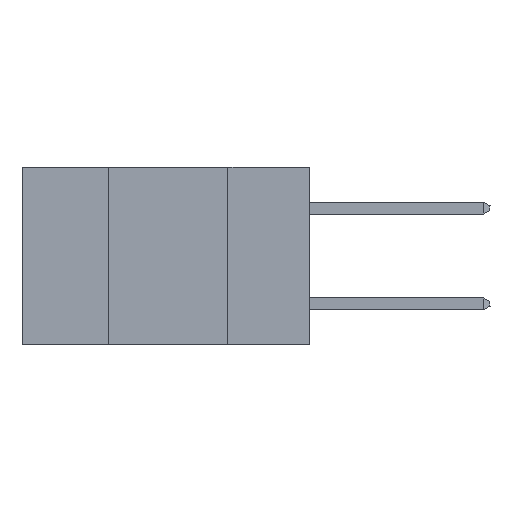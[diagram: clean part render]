
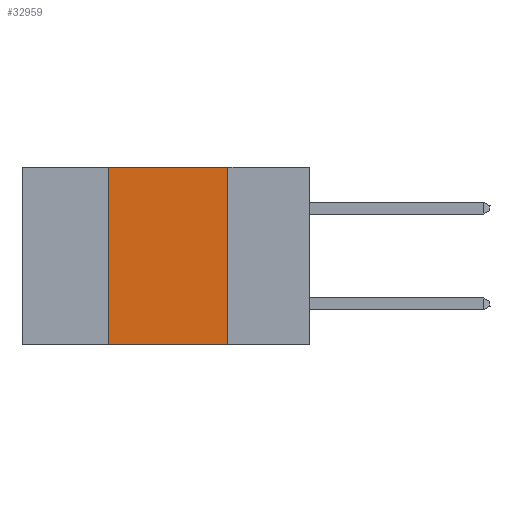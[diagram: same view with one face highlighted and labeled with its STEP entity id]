
A CAD part, left-side view. The second image highlights one B-rep face of the part: STEP entity #32959.
In plain terms, the highlighted planar face has unit normal (-1, 0, 0).
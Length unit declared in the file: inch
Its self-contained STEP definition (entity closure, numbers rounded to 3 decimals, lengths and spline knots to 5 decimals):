
#1785 = FACE_OUTER_BOUND ( 'NONE', #28149, .T. ) ;
#3760 = DIRECTION ( 'NONE',  ( 0., 0., 1. ) ) ;
#4637 = CARTESIAN_POINT ( 'NONE',  ( 0., 0.17, 0. ) ) ;
#5468 = DIRECTION ( 'NONE',  ( 0., -1., 0. ) ) ;
#6344 = CARTESIAN_POINT ( 'NONE',  ( 0., 0.6, -0.37 ) ) ;
#7379 = VERTEX_POINT ( 'NONE', #9560 ) ;
#9560 = CARTESIAN_POINT ( 'NONE',  ( 0., 0.42, 0. ) ) ;
#10012 = VERTEX_POINT ( 'NONE', #13973 ) ;
#13324 = CARTESIAN_POINT ( 'NONE',  ( 0., 0.42, -0.37 ) ) ;
#13857 = ORIENTED_EDGE ( 'NONE', *, *, #39722, .F. ) ;
#13973 = CARTESIAN_POINT ( 'NONE',  ( 0., 0.17, -0.37 ) ) ;
#15135 = CARTESIAN_POINT ( 'NONE',  ( 0., 0.42, 0. ) ) ;
#16659 = LINE ( 'NONE', #4637, #30544 ) ;
#18186 = LINE ( 'NONE', #23768, #26294 ) ;
#18479 = AXIS2_PLACEMENT_3D ( 'NONE', #45113, #23121, #43137 ) ;
#18833 = VERTEX_POINT ( 'NONE', #39176 ) ;
#21761 = VECTOR ( 'NONE', #3760, 39.37008 ) ;
#23121 = DIRECTION ( 'NONE',  ( 1., 0., 0. ) ) ;
#23596 = LINE ( 'NONE', #6344, #42101 ) ;
#23607 = EDGE_CURVE ( 'NONE', #18833, #10012, #16659, .T. ) ;
#23768 = CARTESIAN_POINT ( 'NONE',  ( 0., 0.6, 0. ) ) ;
#25855 = ORIENTED_EDGE ( 'NONE', *, *, #41841, .F. ) ;
#26294 = VECTOR ( 'NONE', #5468, 39.37008 ) ;
#28149 = EDGE_LOOP ( 'NONE', ( #29680, #25855, #13857, #33433 ) ) ;
#29680 = ORIENTED_EDGE ( 'NONE', *, *, #23607, .F. ) ;
#30544 = VECTOR ( 'NONE', #45440, 39.37008 ) ;
#32098 = DIRECTION ( 'NONE',  ( 0., -1., 0. ) ) ;
#32959 = ADVANCED_FACE ( 'NONE', ( #1785 ), #37883, .F. ) ;
#33433 = ORIENTED_EDGE ( 'NONE', *, *, #46192, .T. ) ;
#37883 = PLANE ( 'NONE',  #18479 ) ;
#39176 = CARTESIAN_POINT ( 'NONE',  ( 0., 0.17, 0. ) ) ;
#39722 = EDGE_CURVE ( 'NONE', #46052, #7379, #41415, .T. ) ;
#41415 = LINE ( 'NONE', #15135, #21761 ) ;
#41841 = EDGE_CURVE ( 'NONE', #7379, #18833, #18186, .T. ) ;
#42101 = VECTOR ( 'NONE', #32098, 39.37008 ) ;
#43137 = DIRECTION ( 'NONE',  ( 0., 0., -1. ) ) ;
#45113 = CARTESIAN_POINT ( 'NONE',  ( 0., 0.6, 0. ) ) ;
#45440 = DIRECTION ( 'NONE',  ( 0., 0., -1. ) ) ;
#46052 = VERTEX_POINT ( 'NONE', #13324 ) ;
#46192 = EDGE_CURVE ( 'NONE', #46052, #10012, #23596, .T. ) ;
